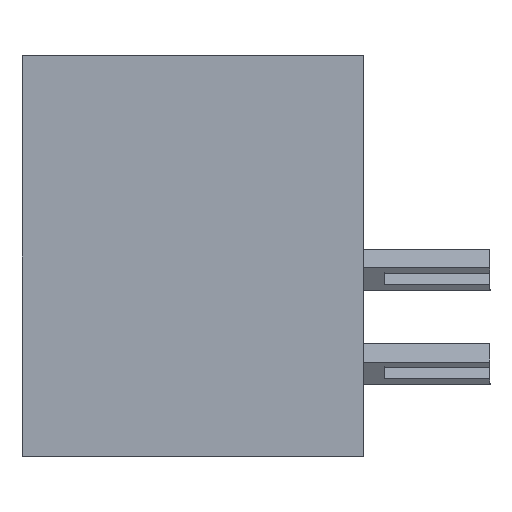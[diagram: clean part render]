
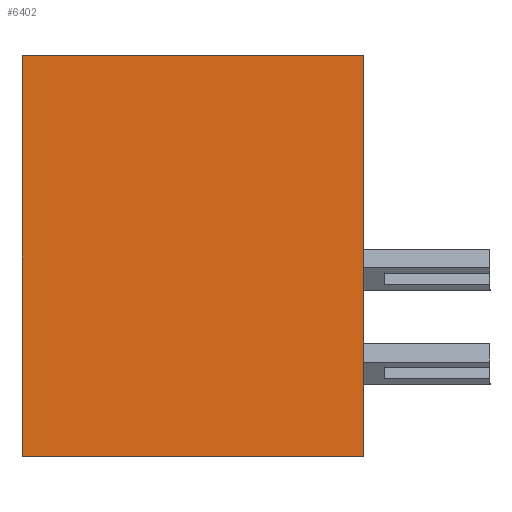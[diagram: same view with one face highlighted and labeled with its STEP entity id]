
A CAD part, left-side view. The second image highlights one B-rep face of the part: STEP entity #6402.
In plain terms, the highlighted planar face has unit normal (-1, 0, 0).
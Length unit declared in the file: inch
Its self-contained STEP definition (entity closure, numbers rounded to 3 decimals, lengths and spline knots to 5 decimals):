
#1448 = DIRECTION ( 'NONE',  ( 0., 0., 1. ) ) ;
#1452 = ORIENTED_EDGE ( 'NONE', *, *, #9880, .F. ) ;
#1471 = EDGE_CURVE ( 'NONE', #12772, #4641, #4296, .T. ) ;
#1542 = AXIS2_PLACEMENT_3D ( 'NONE', #5138, #8799, #9914 ) ;
#2034 = ORIENTED_EDGE ( 'NONE', *, *, #1471, .T. ) ;
#3028 = ORIENTED_EDGE ( 'NONE', *, *, #14768, .T. ) ;
#3195 = CARTESIAN_POINT ( 'NONE',  ( 0., 0., -0.531 ) ) ;
#3463 = EDGE_CURVE ( 'NONE', #12716, #4641, #6342, .T. ) ;
#3859 = VECTOR ( 'NONE', #13911, 39.37008 ) ;
#4020 = VERTEX_POINT ( 'NONE', #5998 ) ;
#4296 = LINE ( 'NONE', #7063, #6211 ) ;
#4558 = DIRECTION ( 'NONE',  ( 0., 0., 1. ) ) ;
#4641 = VERTEX_POINT ( 'NONE', #8353 ) ;
#4671 = DIRECTION ( 'NONE',  ( 0., -1., 0. ) ) ;
#5138 = CARTESIAN_POINT ( 'NONE',  ( 0., 0.453, 0. ) ) ;
#5155 = ORIENTED_EDGE ( 'NONE', *, *, #3463, .F. ) ;
#5368 = CARTESIAN_POINT ( 'NONE',  ( 0., 0.453, 0. ) ) ;
#5430 = CARTESIAN_POINT ( 'NONE',  ( 0., 0.453, 0. ) ) ;
#5998 = CARTESIAN_POINT ( 'NONE',  ( 0., 0.453, -0.531 ) ) ;
#6211 = VECTOR ( 'NONE', #4558, 39.37008 ) ;
#6297 = EDGE_LOOP ( 'NONE', ( #2034, #5155, #1452, #3028 ) ) ;
#6342 = LINE ( 'NONE', #5430, #3859 ) ;
#6402 = ADVANCED_FACE ( 'NONE', ( #7209 ), #8702, .F. ) ;
#6914 = CARTESIAN_POINT ( 'NONE',  ( 0., 0.453, -0.531 ) ) ;
#7063 = CARTESIAN_POINT ( 'NONE',  ( 0., 0., 0. ) ) ;
#7209 = FACE_OUTER_BOUND ( 'NONE', #6297, .T. ) ;
#7254 = VECTOR ( 'NONE', #4671, 39.37008 ) ;
#7655 = LINE ( 'NONE', #12445, #15021 ) ;
#8353 = CARTESIAN_POINT ( 'NONE',  ( 0., 0., 0. ) ) ;
#8702 = PLANE ( 'NONE',  #1542 ) ;
#8799 = DIRECTION ( 'NONE',  ( 1., 0., 0. ) ) ;
#9880 = EDGE_CURVE ( 'NONE', #4020, #12716, #7655, .T. ) ;
#9914 = DIRECTION ( 'NONE',  ( 0., 0., -1. ) ) ;
#10452 = LINE ( 'NONE', #6914, #7254 ) ;
#12445 = CARTESIAN_POINT ( 'NONE',  ( 0., 0.453, 0. ) ) ;
#12716 = VERTEX_POINT ( 'NONE', #5368 ) ;
#12772 = VERTEX_POINT ( 'NONE', #3195 ) ;
#13911 = DIRECTION ( 'NONE',  ( 0., -1., 0. ) ) ;
#14768 = EDGE_CURVE ( 'NONE', #4020, #12772, #10452, .T. ) ;
#15021 = VECTOR ( 'NONE', #1448, 39.37008 ) ;
